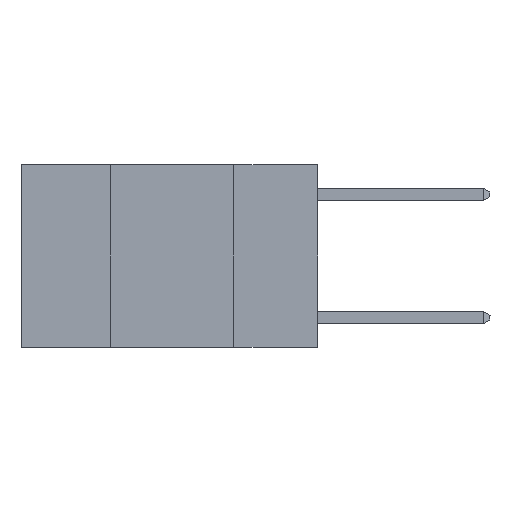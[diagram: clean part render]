
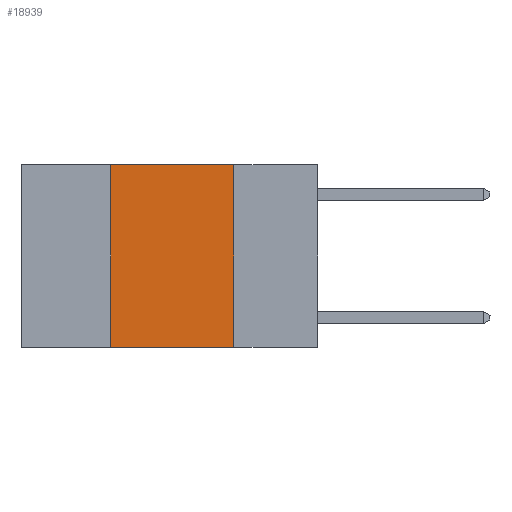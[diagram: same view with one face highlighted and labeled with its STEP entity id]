
A CAD part, left-side view. The second image highlights one B-rep face of the part: STEP entity #18939.
In plain terms, the highlighted planar face has unit normal (-1, 0, 0).
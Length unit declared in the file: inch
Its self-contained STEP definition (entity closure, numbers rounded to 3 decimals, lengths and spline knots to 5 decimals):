
#52 = VECTOR ( 'NONE', #5639, 39.37008 ) ;
#1050 = CARTESIAN_POINT ( 'NONE',  ( 0., 0.42, 0. ) ) ;
#1104 = CARTESIAN_POINT ( 'NONE',  ( 0., 0.42, 0. ) ) ;
#1621 = ORIENTED_EDGE ( 'NONE', *, *, #9192, .F. ) ;
#2847 = LINE ( 'NONE', #3507, #6626 ) ;
#2971 = VECTOR ( 'NONE', #17507, 39.37008 ) ;
#3245 = EDGE_CURVE ( 'NONE', #16245, #3940, #16411, .T. ) ;
#3507 = CARTESIAN_POINT ( 'NONE',  ( 0., 0.17, 0. ) ) ;
#3845 = AXIS2_PLACEMENT_3D ( 'NONE', #18168, #8447, #19804 ) ;
#3940 = VERTEX_POINT ( 'NONE', #11132 ) ;
#5639 = DIRECTION ( 'NONE',  ( 0., -1., 0. ) ) ;
#5891 = ORIENTED_EDGE ( 'NONE', *, *, #10044, .F. ) ;
#5920 = VERTEX_POINT ( 'NONE', #7720 ) ;
#6262 = FACE_OUTER_BOUND ( 'NONE', #11612, .T. ) ;
#6334 = LINE ( 'NONE', #1050, #14478 ) ;
#6457 = CARTESIAN_POINT ( 'NONE',  ( 0., 0.42, -0.37 ) ) ;
#6626 = VECTOR ( 'NONE', #16465, 39.37008 ) ;
#7720 = CARTESIAN_POINT ( 'NONE',  ( 0., 0.17, 0. ) ) ;
#8379 = PLANE ( 'NONE',  #3845 ) ;
#8447 = DIRECTION ( 'NONE',  ( 1., 0., 0. ) ) ;
#9192 = EDGE_CURVE ( 'NONE', #20550, #5920, #9205, .T. ) ;
#9205 = LINE ( 'NONE', #18581, #52 ) ;
#10044 = EDGE_CURVE ( 'NONE', #16245, #20550, #6334, .T. ) ;
#11132 = CARTESIAN_POINT ( 'NONE',  ( 0., 0.17, -0.37 ) ) ;
#11612 = EDGE_LOOP ( 'NONE', ( #18355, #1621, #5891, #18878 ) ) ;
#12398 = DIRECTION ( 'NONE',  ( 0., 0., 1. ) ) ;
#12639 = CARTESIAN_POINT ( 'NONE',  ( 0., 0.6, -0.37 ) ) ;
#14478 = VECTOR ( 'NONE', #12398, 39.37008 ) ;
#16245 = VERTEX_POINT ( 'NONE', #6457 ) ;
#16365 = EDGE_CURVE ( 'NONE', #5920, #3940, #2847, .T. ) ;
#16411 = LINE ( 'NONE', #12639, #2971 ) ;
#16465 = DIRECTION ( 'NONE',  ( 0., 0., -1. ) ) ;
#17507 = DIRECTION ( 'NONE',  ( 0., -1., 0. ) ) ;
#18168 = CARTESIAN_POINT ( 'NONE',  ( 0., 0.6, 0. ) ) ;
#18355 = ORIENTED_EDGE ( 'NONE', *, *, #16365, .F. ) ;
#18581 = CARTESIAN_POINT ( 'NONE',  ( 0., 0.6, 0. ) ) ;
#18878 = ORIENTED_EDGE ( 'NONE', *, *, #3245, .T. ) ;
#18939 = ADVANCED_FACE ( 'NONE', ( #6262 ), #8379, .F. ) ;
#19804 = DIRECTION ( 'NONE',  ( 0., 0., -1. ) ) ;
#20550 = VERTEX_POINT ( 'NONE', #1104 ) ;
